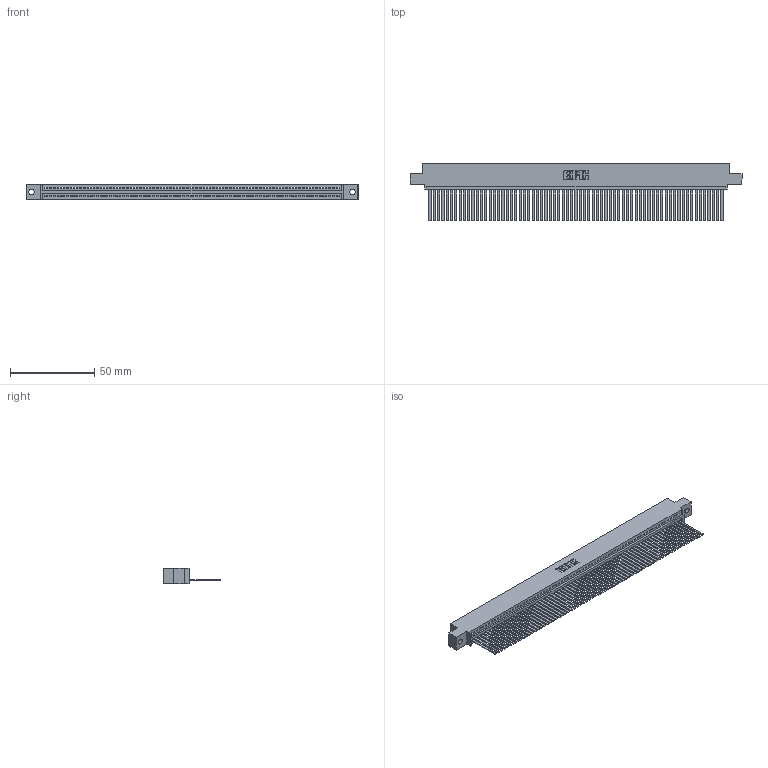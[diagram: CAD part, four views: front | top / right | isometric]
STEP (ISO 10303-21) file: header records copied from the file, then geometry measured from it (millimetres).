
FILE_DESCRIPTION (( 'STEP AP203' ), '1' );
FILE_NAME ('345-069-544-402.STEP', '2018-09-30T20:01:12', ( '' ), ( '' ), 'SwSTEP 2.0', 'SolidWorks 2016', '' );
FILE_SCHEMA (( 'CONFIG_CONTROL_DESIGN' ));
Length unit declared in the file: inch
Products named in the file (3): 345-069-544-402; 345-292-001_345-293-144; 345 Part_0.110 Offset - 0.128 Dia
Assembly tree (70 placements, depth 2):
  345-069-544-402
    345 Part_0.110 Offset - 0.128 Dia
    345-292-001_345-293-144  x69
Bounding box: 196.47 x 33.96 x 9.4 mm (x, y, z)
Volume: 19571.1 mm3; surface area: 28584.5 mm2
Topology: 70 solids, 70 shells, 3718 faces, 11255 edges, 7410 vertices
Faces by surface type: plane 2568, cylinder 1150
Entity records: 48247 total; most frequent: ORIENTED_EDGE 8366, CARTESIAN_POINT 8363, DIRECTION 7261, EDGE_CURVE 4183, LINE 3779, VECTOR 3779, VERTEX_POINT 2786, AXIS2_PLACEMENT_3D 1741
